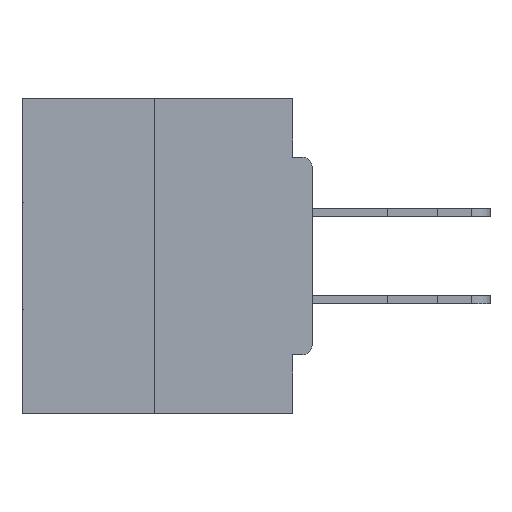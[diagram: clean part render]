
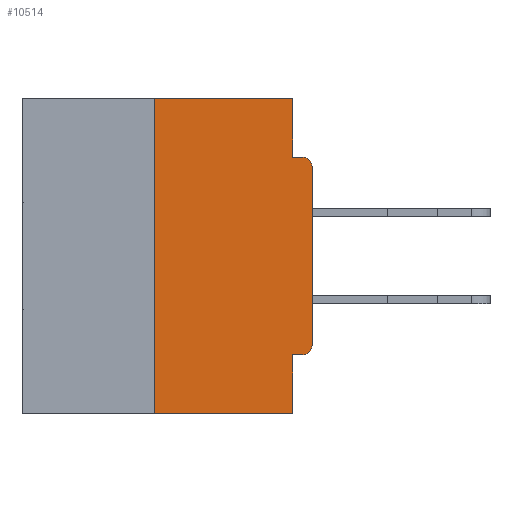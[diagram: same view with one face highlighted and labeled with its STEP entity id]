
A CAD part, left-side view. The second image highlights one B-rep face of the part: STEP entity #10514.
In plain terms, the highlighted planar face has unit normal (-1, 0, 0).
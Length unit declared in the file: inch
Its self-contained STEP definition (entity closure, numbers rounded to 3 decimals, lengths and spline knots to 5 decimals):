
#378 = VERTEX_POINT ( 'NONE', #39556 ) ;
#1313 = CARTESIAN_POINT ( 'NONE',  ( 0., 0.031, 0. ) ) ;
#2590 = PLANE ( 'NONE',  #36081 ) ;
#2752 = CARTESIAN_POINT ( 'NONE',  ( 0., 0.031, -0.5 ) ) ;
#3422 = VERTEX_POINT ( 'NONE', #17481 ) ;
#3538 = VECTOR ( 'NONE', #16639, 39.37008 ) ;
#4359 = EDGE_CURVE ( 'NONE', #36701, #24202, #29420, .T. ) ;
#4890 = EDGE_CURVE ( 'NONE', #36870, #24102, #11189, .T. ) ;
#5460 = DIRECTION ( 'NONE',  ( 0., 0., -1. ) ) ;
#7451 = CARTESIAN_POINT ( 'NONE',  ( 0., 0., -0.0935 ) ) ;
#7475 = EDGE_CURVE ( 'NONE', #37981, #36701, #28797, .T. ) ;
#8334 = VECTOR ( 'NONE', #36997, 39.37008 ) ;
#8991 = AXIS2_PLACEMENT_3D ( 'NONE', #12925, #19035, #9733 ) ;
#8995 = VECTOR ( 'NONE', #36782, 39.37008 ) ;
#9733 = DIRECTION ( 'NONE',  ( 0., 0., -1. ) ) ;
#10243 = VECTOR ( 'NONE', #15230, 39.37008 ) ;
#10514 = ADVANCED_FACE ( 'NONE', ( #17073 ), #2590, .F. ) ;
#10921 = DIRECTION ( 'NONE',  ( 0., 0., -1. ) ) ;
#11189 = LINE ( 'NONE', #12166, #10243 ) ;
#11352 = ORIENTED_EDGE ( 'NONE', *, *, #7475, .F. ) ;
#11457 = CIRCLE ( 'NONE', #8991, 0.015 ) ;
#11796 = DIRECTION ( 'NONE',  ( 0., -1., 0. ) ) ;
#12166 = CARTESIAN_POINT ( 'NONE',  ( 0., 0., -0.4065 ) ) ;
#12242 = ORIENTED_EDGE ( 'NONE', *, *, #13322, .T. ) ;
#12925 = CARTESIAN_POINT ( 'NONE',  ( 0., 0.015, -0.1085 ) ) ;
#13322 = EDGE_CURVE ( 'NONE', #37981, #30112, #28025, .T. ) ;
#15230 = DIRECTION ( 'NONE',  ( 0., 1., 0. ) ) ;
#15723 = VECTOR ( 'NONE', #5460, 39.37008 ) ;
#16182 = CARTESIAN_POINT ( 'NONE',  ( 0., 0.031, -0.5 ) ) ;
#16556 = ORIENTED_EDGE ( 'NONE', *, *, #36666, .F. ) ;
#16639 = DIRECTION ( 'NONE',  ( 0., -1., 0. ) ) ;
#16937 = ORIENTED_EDGE ( 'NONE', *, *, #31913, .F. ) ;
#17073 = FACE_OUTER_BOUND ( 'NONE', #37549, .T. ) ;
#17080 = CARTESIAN_POINT ( 'NONE',  ( 0., 0.25, -0.5 ) ) ;
#17481 = CARTESIAN_POINT ( 'NONE',  ( 0., 0.015, -0.0935 ) ) ;
#19035 = DIRECTION ( 'NONE',  ( -1., 0., 0. ) ) ;
#19479 = LINE ( 'NONE', #25058, #8995 ) ;
#19713 = CARTESIAN_POINT ( 'NONE',  ( 0., 0.031, -0.4065 ) ) ;
#20333 = VECTOR ( 'NONE', #11796, 39.37008 ) ;
#20355 = ORIENTED_EDGE ( 'NONE', *, *, #32069, .T. ) ;
#21473 = CARTESIAN_POINT ( 'NONE',  ( 0., 0.46, -0.5 ) ) ;
#21739 = AXIS2_PLACEMENT_3D ( 'NONE', #26739, #33061, #23512 ) ;
#21859 = VECTOR ( 'NONE', #25915, 39.37008 ) ;
#21891 = ORIENTED_EDGE ( 'NONE', *, *, #4359, .F. ) ;
#22905 = CARTESIAN_POINT ( 'NONE',  ( 0., 0.25, 0. ) ) ;
#23148 = CARTESIAN_POINT ( 'NONE',  ( 0., 0., -0.3915 ) ) ;
#23154 = DIRECTION ( 'NONE',  ( 0., 0., 1. ) ) ;
#23192 = ORIENTED_EDGE ( 'NONE', *, *, #23231, .T. ) ;
#23231 = EDGE_CURVE ( 'NONE', #36870, #39342, #24547, .T. ) ;
#23512 = DIRECTION ( 'NONE',  ( 0., 0., -1. ) ) ;
#23679 = ORIENTED_EDGE ( 'NONE', *, *, #32263, .F. ) ;
#24102 = VERTEX_POINT ( 'NONE', #19713 ) ;
#24202 = VERTEX_POINT ( 'NONE', #38922 ) ;
#24547 = CIRCLE ( 'NONE', #21739, 0.015 ) ;
#25058 = CARTESIAN_POINT ( 'NONE',  ( 0., 0., 0. ) ) ;
#25915 = DIRECTION ( 'NONE',  ( 0., 0., -1. ) ) ;
#26739 = CARTESIAN_POINT ( 'NONE',  ( 0., 0.015, -0.3915 ) ) ;
#26820 = VECTOR ( 'NONE', #23154, 39.37008 ) ;
#28025 = LINE ( 'NONE', #21473, #20333 ) ;
#28797 = LINE ( 'NONE', #35277, #26820 ) ;
#29420 = LINE ( 'NONE', #36863, #8334 ) ;
#29470 = CARTESIAN_POINT ( 'NONE',  ( 0., 0.46, 0. ) ) ;
#30026 = ORIENTED_EDGE ( 'NONE', *, *, #4890, .F. ) ;
#30027 = LINE ( 'NONE', #1313, #21859 ) ;
#30112 = VERTEX_POINT ( 'NONE', #2752 ) ;
#30271 = VERTEX_POINT ( 'NONE', #36367 ) ;
#30548 = EDGE_CURVE ( 'NONE', #378, #3422, #11457, .T. ) ;
#30832 = LINE ( 'NONE', #7451, #3538 ) ;
#31913 = EDGE_CURVE ( 'NONE', #24102, #30112, #32949, .T. ) ;
#32069 = EDGE_CURVE ( 'NONE', #39342, #378, #19479, .T. ) ;
#32263 = EDGE_CURVE ( 'NONE', #24202, #30271, #30027, .T. ) ;
#32949 = LINE ( 'NONE', #16182, #15723 ) ;
#33061 = DIRECTION ( 'NONE',  ( -1., 0., 0. ) ) ;
#35169 = ORIENTED_EDGE ( 'NONE', *, *, #30548, .T. ) ;
#35277 = CARTESIAN_POINT ( 'NONE',  ( 0., 0.25, 0. ) ) ;
#36081 = AXIS2_PLACEMENT_3D ( 'NONE', #29470, #38882, #10921 ) ;
#36367 = CARTESIAN_POINT ( 'NONE',  ( 0., 0.031, -0.0935 ) ) ;
#36448 = CARTESIAN_POINT ( 'NONE',  ( 0., 0.015, -0.4065 ) ) ;
#36666 = EDGE_CURVE ( 'NONE', #30271, #3422, #30832, .T. ) ;
#36701 = VERTEX_POINT ( 'NONE', #22905 ) ;
#36782 = DIRECTION ( 'NONE',  ( 0., 0., 1. ) ) ;
#36863 = CARTESIAN_POINT ( 'NONE',  ( 0., 0.46, 0. ) ) ;
#36870 = VERTEX_POINT ( 'NONE', #36448 ) ;
#36997 = DIRECTION ( 'NONE',  ( 0., -1., 0. ) ) ;
#37549 = EDGE_LOOP ( 'NONE', ( #21891, #11352, #12242, #16937, #30026, #23192, #20355, #35169, #16556, #23679 ) ) ;
#37981 = VERTEX_POINT ( 'NONE', #17080 ) ;
#38882 = DIRECTION ( 'NONE',  ( 1., 0., 0. ) ) ;
#38922 = CARTESIAN_POINT ( 'NONE',  ( 0., 0.031, 0. ) ) ;
#39342 = VERTEX_POINT ( 'NONE', #23148 ) ;
#39556 = CARTESIAN_POINT ( 'NONE',  ( 0., 0., -0.1085 ) ) ;
